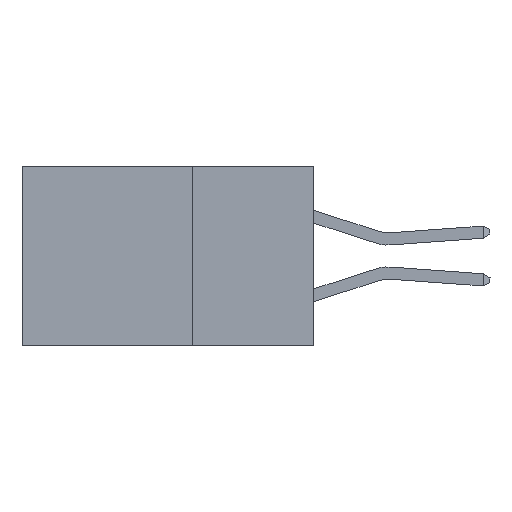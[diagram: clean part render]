
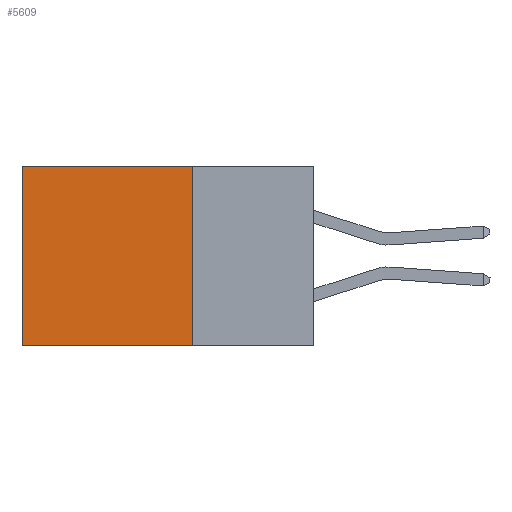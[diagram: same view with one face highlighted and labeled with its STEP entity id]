
A CAD part, left-side view. The second image highlights one B-rep face of the part: STEP entity #5609.
In plain terms, the highlighted planar face has unit normal (-1, 0, 0).
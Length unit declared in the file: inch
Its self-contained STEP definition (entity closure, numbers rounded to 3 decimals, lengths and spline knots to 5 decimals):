
#106 = ORIENTED_EDGE ( 'NONE', *, *, #26358, .T. ) ;
#949 = DIRECTION ( 'NONE',  ( 0., 1., 0. ) ) ;
#1135 = CARTESIAN_POINT ( 'NONE',  ( 0.2875, 0.25, 0. ) ) ;
#1351 = PLANE ( 'NONE',  #6091 ) ;
#2130 = CARTESIAN_POINT ( 'NONE',  ( 0.2875, 0.25, -0.37 ) ) ;
#3779 = EDGE_CURVE ( 'NONE', #29121, #23854, #8427, .T. ) ;
#3839 = DIRECTION ( 'NONE',  ( 0., 0., -1. ) ) ;
#4376 = VECTOR ( 'NONE', #949, 39.37008 ) ;
#5514 = ORIENTED_EDGE ( 'NONE', *, *, #19428, .F. ) ;
#5609 = ADVANCED_FACE ( 'NONE', ( #6573 ), #1351, .F. ) ;
#5949 = ORIENTED_EDGE ( 'NONE', *, *, #20298, .T. ) ;
#6047 = CARTESIAN_POINT ( 'NONE',  ( 0.2875, 0.6, 0. ) ) ;
#6091 = AXIS2_PLACEMENT_3D ( 'NONE', #1135, #25687, #3839 ) ;
#6573 = FACE_OUTER_BOUND ( 'NONE', #14406, .T. ) ;
#6674 = LINE ( 'NONE', #2130, #10527 ) ;
#8427 = LINE ( 'NONE', #24520, #9981 ) ;
#9378 = CARTESIAN_POINT ( 'NONE',  ( 0.2875, 0.6, -0.37 ) ) ;
#9755 = VECTOR ( 'NONE', #16077, 39.37008 ) ;
#9981 = VECTOR ( 'NONE', #29031, 39.37008 ) ;
#10527 = VECTOR ( 'NONE', #13900, 39.37008 ) ;
#11184 = CARTESIAN_POINT ( 'NONE',  ( 0.2875, 0.25, 0. ) ) ;
#11861 = VERTEX_POINT ( 'NONE', #6047 ) ;
#13900 = DIRECTION ( 'NONE',  ( 0., 1., 0. ) ) ;
#14240 = CARTESIAN_POINT ( 'NONE',  ( 0.2875, 0.25, 0. ) ) ;
#14406 = EDGE_LOOP ( 'NONE', ( #106, #5514, #20588, #5949 ) ) ;
#16077 = DIRECTION ( 'NONE',  ( 0., 0., -1. ) ) ;
#17765 = LINE ( 'NONE', #30750, #9755 ) ;
#19428 = EDGE_CURVE ( 'NONE', #23854, #23392, #6674, .T. ) ;
#20298 = EDGE_CURVE ( 'NONE', #29121, #11861, #29675, .T. ) ;
#20588 = ORIENTED_EDGE ( 'NONE', *, *, #3779, .F. ) ;
#23392 = VERTEX_POINT ( 'NONE', #9378 ) ;
#23756 = CARTESIAN_POINT ( 'NONE',  ( 0.2875, 0.25, -0.37 ) ) ;
#23854 = VERTEX_POINT ( 'NONE', #23756 ) ;
#24520 = CARTESIAN_POINT ( 'NONE',  ( 0.2875, 0.25, 0. ) ) ;
#25687 = DIRECTION ( 'NONE',  ( 1., 0., 0. ) ) ;
#26358 = EDGE_CURVE ( 'NONE', #11861, #23392, #17765, .T. ) ;
#29031 = DIRECTION ( 'NONE',  ( 0., 0., -1. ) ) ;
#29121 = VERTEX_POINT ( 'NONE', #14240 ) ;
#29675 = LINE ( 'NONE', #11184, #4376 ) ;
#30750 = CARTESIAN_POINT ( 'NONE',  ( 0.2875, 0.6, 0. ) ) ;
